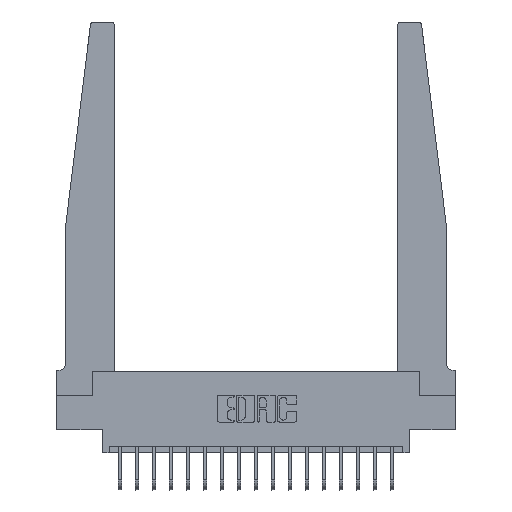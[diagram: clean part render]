
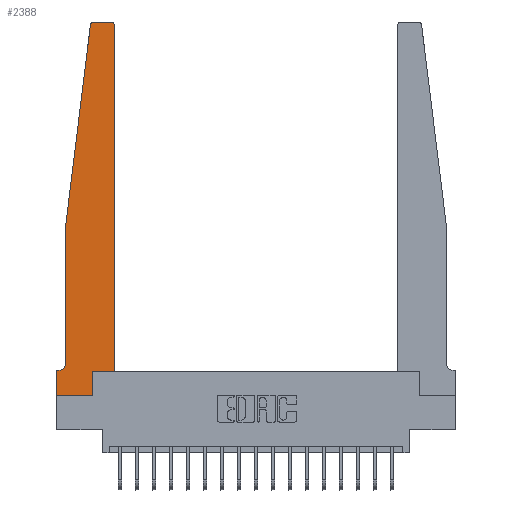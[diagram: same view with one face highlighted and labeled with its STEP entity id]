
A CAD part, top view. The second image highlights one B-rep face of the part: STEP entity #2388.
In plain terms, the highlighted planar face has unit normal (0, 0, 1).
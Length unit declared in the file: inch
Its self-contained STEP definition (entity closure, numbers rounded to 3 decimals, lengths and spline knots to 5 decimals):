
#649 = CARTESIAN_POINT ( 'NONE',  ( 0.395, 2.75, 0.37 ) ) ;
#881 = CARTESIAN_POINT ( 'NONE',  ( 0.27653, 2.75, 0.37 ) ) ;
#1204 = AXIS2_PLACEMENT_3D ( 'NONE', #18534, #5316, #1919 ) ;
#1276 = LINE ( 'NONE', #8070, #19694 ) ;
#1489 = DIRECTION ( 'NONE',  ( 0., -1., 0. ) ) ;
#1579 = VECTOR ( 'NONE', #3378, 39.37008 ) ;
#1919 = DIRECTION ( 'NONE',  ( -1., 0., 0. ) ) ;
#2125 = CARTESIAN_POINT ( 'NONE',  ( 0.065, 1.25, 0.37 ) ) ;
#2388 = ADVANCED_FACE ( 'NONE', ( #20101 ), #12563, .T. ) ;
#2536 = AXIS2_PLACEMENT_3D ( 'NONE', #3667, #7068, #5093 ) ;
#2581 = CARTESIAN_POINT ( 'NONE',  ( 0., 0.1875, 0.37 ) ) ;
#2804 = EDGE_CURVE ( 'NONE', #18959, #17042, #12538, .T. ) ;
#3198 = CARTESIAN_POINT ( 'NONE',  ( 0., 0., 0.37 ) ) ;
#3233 = EDGE_CURVE ( 'NONE', #17042, #18902, #5287, .T. ) ;
#3318 = ORIENTED_EDGE ( 'NONE', *, *, #17792, .T. ) ;
#3356 = ORIENTED_EDGE ( 'NONE', *, *, #2804, .T. ) ;
#3378 = DIRECTION ( 'NONE',  ( 0., 1., 0. ) ) ;
#3396 = CARTESIAN_POINT ( 'NONE',  ( 0.24675, 2.72367, 0.37 ) ) ;
#3643 = EDGE_CURVE ( 'NONE', #13982, #4229, #13696, .T. ) ;
#3667 = CARTESIAN_POINT ( 'NONE',  ( 0.27653, 2.72, 0.37 ) ) ;
#3788 = DIRECTION ( 'NONE',  ( -0.122, -0.992, 0. ) ) ;
#3853 = DIRECTION ( 'NONE',  ( 0., 0., 1. ) ) ;
#3856 = CARTESIAN_POINT ( 'NONE',  ( 0.425, 2.72, 0.37 ) ) ;
#4081 = VECTOR ( 'NONE', #8652, 39.37008 ) ;
#4194 = LINE ( 'NONE', #9332, #6223 ) ;
#4229 = VERTEX_POINT ( 'NONE', #15142 ) ;
#4439 = CARTESIAN_POINT ( 'NONE',  ( 0.425, 0.18, 0.37 ) ) ;
#4484 = VECTOR ( 'NONE', #12667, 39.37008 ) ;
#4822 = ORIENTED_EDGE ( 'NONE', *, *, #6695, .T. ) ;
#4929 = VERTEX_POINT ( 'NONE', #16172 ) ;
#5093 = DIRECTION ( 'NONE',  ( 1., 0., 0. ) ) ;
#5287 = CIRCLE ( 'NONE', #15420, 0.03 ) ;
#5316 = DIRECTION ( 'NONE',  ( 0., 0., -1. ) ) ;
#5386 = DIRECTION ( 'NONE',  ( 1., 0., 0. ) ) ;
#5462 = VECTOR ( 'NONE', #3788, 39.37008 ) ;
#5519 = DIRECTION ( 'NONE',  ( 0., 1., 0. ) ) ;
#5708 = CARTESIAN_POINT ( 'NONE',  ( 0.065, 1.25, 0.37 ) ) ;
#6085 = VERTEX_POINT ( 'NONE', #15982 ) ;
#6223 = VECTOR ( 'NONE', #14260, 39.37008 ) ;
#6447 = EDGE_CURVE ( 'NONE', #11965, #4929, #1276, .T. ) ;
#6695 = EDGE_CURVE ( 'NONE', #4929, #18723, #11368, .T. ) ;
#6864 = LINE ( 'NONE', #2125, #5462 ) ;
#7068 = DIRECTION ( 'NONE',  ( 0., 0., 1. ) ) ;
#7094 = CIRCLE ( 'NONE', #2536, 0.03 ) ;
#7852 = EDGE_CURVE ( 'NONE', #6085, #15582, #10281, .T. ) ;
#8070 = CARTESIAN_POINT ( 'NONE',  ( 0.065, 1.25, 0.37 ) ) ;
#8515 = EDGE_CURVE ( 'NONE', #18781, #11965, #6864, .T. ) ;
#8652 = DIRECTION ( 'NONE',  ( 0., -1., 0. ) ) ;
#8867 = CARTESIAN_POINT ( 'NONE',  ( 0., 0., 0.37 ) ) ;
#9134 = CARTESIAN_POINT ( 'NONE',  ( 0.425, 0.18, 0.37 ) ) ;
#9159 = DIRECTION ( 'NONE',  ( 0., 0., 1. ) ) ;
#9301 = CARTESIAN_POINT ( 'NONE',  ( 0., 0.1875, 0.37 ) ) ;
#9332 = CARTESIAN_POINT ( 'NONE',  ( 0.065, 0.1875, 0.37 ) ) ;
#10224 = EDGE_CURVE ( 'NONE', #18723, #13982, #4194, .T. ) ;
#10245 = LINE ( 'NONE', #16785, #18928 ) ;
#10281 = LINE ( 'NONE', #20306, #1579 ) ;
#10296 = CARTESIAN_POINT ( 'NONE',  ( 0.015, 0.1875, 0.37 ) ) ;
#11125 = EDGE_CURVE ( 'NONE', #15582, #18959, #14184, .T. ) ;
#11368 = CIRCLE ( 'NONE', #1204, 0.05 ) ;
#11965 = VERTEX_POINT ( 'NONE', #5708 ) ;
#12008 = VERTEX_POINT ( 'NONE', #881 ) ;
#12058 = DIRECTION ( 'NONE',  ( 1., 0., 0. ) ) ;
#12538 = LINE ( 'NONE', #9134, #16421 ) ;
#12563 = PLANE ( 'NONE',  #18587 ) ;
#12604 = VECTOR ( 'NONE', #21111, 39.37008 ) ;
#12667 = DIRECTION ( 'NONE',  ( 1., 0., 0. ) ) ;
#13696 = LINE ( 'NONE', #8867, #4081 ) ;
#13754 = EDGE_LOOP ( 'NONE', ( #16800, #3318, #19999, #16244, #4822, #16040, #17416, #18815, #19030, #20030, #3356, #14728 ) ) ;
#13982 = VERTEX_POINT ( 'NONE', #9301 ) ;
#14184 = LINE ( 'NONE', #4439, #4484 ) ;
#14260 = DIRECTION ( 'NONE',  ( -1., 0., 0. ) ) ;
#14480 = LINE ( 'NONE', #3198, #12604 ) ;
#14728 = ORIENTED_EDGE ( 'NONE', *, *, #3233, .T. ) ;
#15037 = EDGE_CURVE ( 'NONE', #4229, #6085, #14480, .T. ) ;
#15142 = CARTESIAN_POINT ( 'NONE',  ( 0., 0., 0.37 ) ) ;
#15420 = AXIS2_PLACEMENT_3D ( 'NONE', #20445, #3853, #5386 ) ;
#15582 = VERTEX_POINT ( 'NONE', #21087 ) ;
#15982 = CARTESIAN_POINT ( 'NONE',  ( 0.2605, 0., 0.37 ) ) ;
#16040 = ORIENTED_EDGE ( 'NONE', *, *, #10224, .T. ) ;
#16172 = CARTESIAN_POINT ( 'NONE',  ( 0.065, 0.2375, 0.37 ) ) ;
#16244 = ORIENTED_EDGE ( 'NONE', *, *, #6447, .T. ) ;
#16421 = VECTOR ( 'NONE', #5519, 39.37008 ) ;
#16785 = CARTESIAN_POINT ( 'NONE',  ( 0.25, 2.75, 0.37 ) ) ;
#16800 = ORIENTED_EDGE ( 'NONE', *, *, #17784, .T. ) ;
#16896 = DIRECTION ( 'NONE',  ( -1., 0., 0. ) ) ;
#17042 = VERTEX_POINT ( 'NONE', #3856 ) ;
#17416 = ORIENTED_EDGE ( 'NONE', *, *, #3643, .T. ) ;
#17696 = CARTESIAN_POINT ( 'NONE',  ( 0.425, 0.18, 0.37 ) ) ;
#17784 = EDGE_CURVE ( 'NONE', #18902, #12008, #10245, .T. ) ;
#17792 = EDGE_CURVE ( 'NONE', #12008, #18781, #7094, .T. ) ;
#18534 = CARTESIAN_POINT ( 'NONE',  ( 0.015, 0.2375, 0.37 ) ) ;
#18587 = AXIS2_PLACEMENT_3D ( 'NONE', #2581, #9159, #12058 ) ;
#18723 = VERTEX_POINT ( 'NONE', #10296 ) ;
#18781 = VERTEX_POINT ( 'NONE', #3396 ) ;
#18815 = ORIENTED_EDGE ( 'NONE', *, *, #15037, .T. ) ;
#18902 = VERTEX_POINT ( 'NONE', #649 ) ;
#18928 = VECTOR ( 'NONE', #16896, 39.37008 ) ;
#18959 = VERTEX_POINT ( 'NONE', #17696 ) ;
#19030 = ORIENTED_EDGE ( 'NONE', *, *, #7852, .T. ) ;
#19694 = VECTOR ( 'NONE', #1489, 39.37008 ) ;
#19999 = ORIENTED_EDGE ( 'NONE', *, *, #8515, .T. ) ;
#20030 = ORIENTED_EDGE ( 'NONE', *, *, #11125, .T. ) ;
#20101 = FACE_OUTER_BOUND ( 'NONE', #13754, .T. ) ;
#20306 = CARTESIAN_POINT ( 'NONE',  ( 0.2605, 0.18, 0.37 ) ) ;
#20445 = CARTESIAN_POINT ( 'NONE',  ( 0.395, 2.72, 0.37 ) ) ;
#21087 = CARTESIAN_POINT ( 'NONE',  ( 0.2605, 0.18, 0.37 ) ) ;
#21111 = DIRECTION ( 'NONE',  ( 1., 0., 0. ) ) ;
